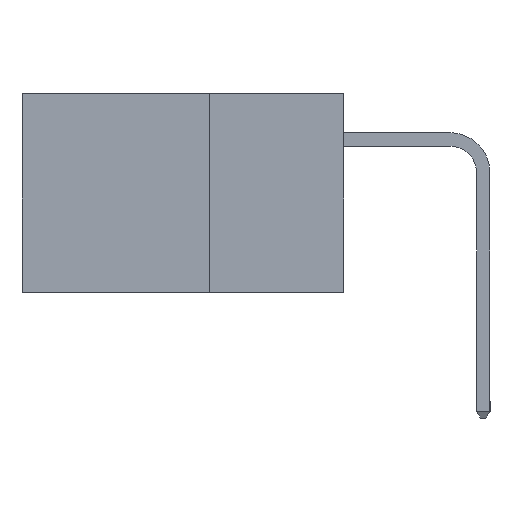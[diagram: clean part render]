
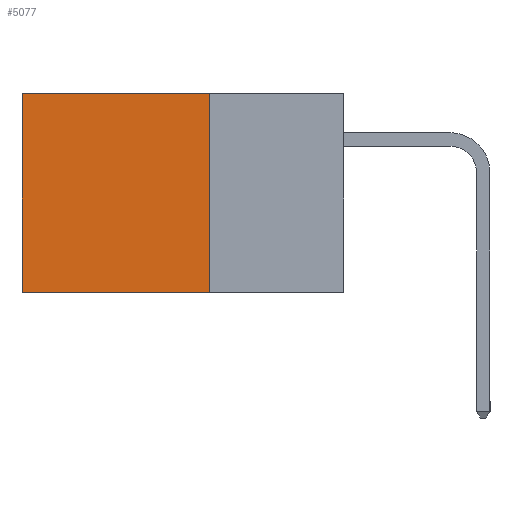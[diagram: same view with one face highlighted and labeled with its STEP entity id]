
A CAD part, left-side view. The second image highlights one B-rep face of the part: STEP entity #5077.
In plain terms, the highlighted planar face has unit normal (-1, 0, 0).
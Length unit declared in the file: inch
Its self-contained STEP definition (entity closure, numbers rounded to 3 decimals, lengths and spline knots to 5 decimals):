
#213 = CARTESIAN_POINT ( 'NONE',  ( 0.2615, 0.6, -0.37 ) ) ;
#667 = CARTESIAN_POINT ( 'NONE',  ( 0.2615, 0.25, -0.37 ) ) ;
#1421 = VERTEX_POINT ( 'NONE', #5853 ) ;
#1736 = CARTESIAN_POINT ( 'NONE',  ( 0.2615, 0.25, -0.37 ) ) ;
#2342 = AXIS2_PLACEMENT_3D ( 'NONE', #14778, #14715, #14693 ) ;
#2814 = VECTOR ( 'NONE', #18516, 39.37008 ) ;
#3044 = EDGE_CURVE ( 'NONE', #13944, #13467, #17997, .T. ) ;
#3048 = EDGE_CURVE ( 'NONE', #6114, #1421, #17579, .T. ) ;
#3192 = DIRECTION ( 'NONE',  ( 0., 1., 0. ) ) ;
#3841 = CARTESIAN_POINT ( 'NONE',  ( 0.2615, 0.6, 0. ) ) ;
#4804 = VECTOR ( 'NONE', #3192, 39.37008 ) ;
#5077 = ADVANCED_FACE ( 'NONE', ( #7083 ), #14754, .F. ) ;
#5853 = CARTESIAN_POINT ( 'NONE',  ( 0.2615, 0.6, -0.37 ) ) ;
#6114 = VERTEX_POINT ( 'NONE', #3841 ) ;
#6715 = ORIENTED_EDGE ( 'NONE', *, *, #3048, .T. ) ;
#7083 = FACE_OUTER_BOUND ( 'NONE', #16205, .T. ) ;
#7889 = CARTESIAN_POINT ( 'NONE',  ( 0.2615, 0.25, 0. ) ) ;
#10224 = ORIENTED_EDGE ( 'NONE', *, *, #14456, .F. ) ;
#10906 = CARTESIAN_POINT ( 'NONE',  ( 0.2615, 0.25, -0.37 ) ) ;
#11327 = CARTESIAN_POINT ( 'NONE',  ( 0.2615, 0.25, 0. ) ) ;
#11979 = LINE ( 'NONE', #11327, #14867 ) ;
#12455 = LINE ( 'NONE', #1736, #4804 ) ;
#12744 = DIRECTION ( 'NONE',  ( 0., 1., 0. ) ) ;
#13467 = VERTEX_POINT ( 'NONE', #10906 ) ;
#13871 = VECTOR ( 'NONE', #15355, 39.37008 ) ;
#13944 = VERTEX_POINT ( 'NONE', #7889 ) ;
#14456 = EDGE_CURVE ( 'NONE', #13467, #1421, #12455, .T. ) ;
#14693 = DIRECTION ( 'NONE',  ( 0., 0., -1. ) ) ;
#14715 = DIRECTION ( 'NONE',  ( 1., 0., 0. ) ) ;
#14754 = PLANE ( 'NONE',  #2342 ) ;
#14778 = CARTESIAN_POINT ( 'NONE',  ( 0.2615, 0.25, -0.37 ) ) ;
#14867 = VECTOR ( 'NONE', #12744, 39.37008 ) ;
#15355 = DIRECTION ( 'NONE',  ( 0., 0., -1. ) ) ;
#15954 = ORIENTED_EDGE ( 'NONE', *, *, #3044, .F. ) ;
#15965 = EDGE_CURVE ( 'NONE', #13944, #6114, #11979, .T. ) ;
#16205 = EDGE_LOOP ( 'NONE', ( #6715, #10224, #15954, #18038 ) ) ;
#17579 = LINE ( 'NONE', #213, #2814 ) ;
#17997 = LINE ( 'NONE', #667, #13871 ) ;
#18038 = ORIENTED_EDGE ( 'NONE', *, *, #15965, .T. ) ;
#18516 = DIRECTION ( 'NONE',  ( 0., 0., -1. ) ) ;
